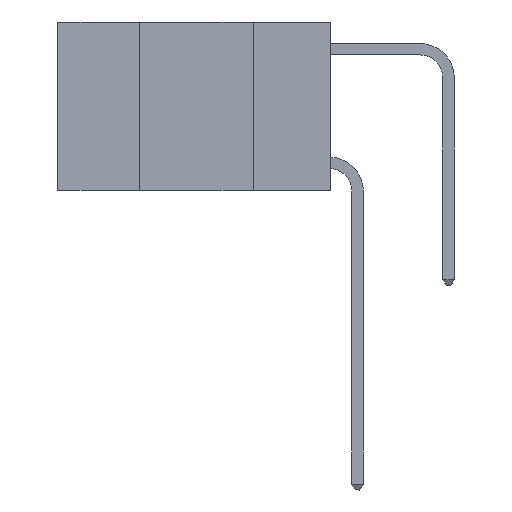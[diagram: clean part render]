
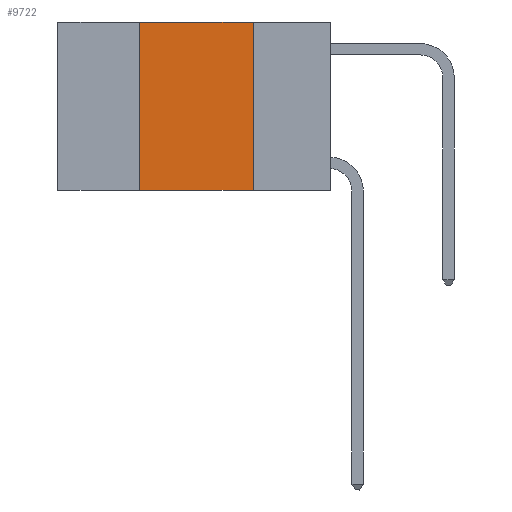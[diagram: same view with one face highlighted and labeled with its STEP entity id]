
A CAD part, left-side view. The second image highlights one B-rep face of the part: STEP entity #9722.
In plain terms, the highlighted planar face has unit normal (-1, 0, 0).
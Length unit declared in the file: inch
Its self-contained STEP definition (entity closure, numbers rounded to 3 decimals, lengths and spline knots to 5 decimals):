
#338 = ORIENTED_EDGE ( 'NONE', *, *, #16720, .T. ) ;
#473 = CARTESIAN_POINT ( 'NONE',  ( 0., 0.6, 0. ) ) ;
#1510 = CARTESIAN_POINT ( 'NONE',  ( 0., 0.6, -0.37 ) ) ;
#2065 = PLANE ( 'NONE',  #4642 ) ;
#2430 = CARTESIAN_POINT ( 'NONE',  ( 0., 0.6, 0. ) ) ;
#2546 = LINE ( 'NONE', #13820, #17581 ) ;
#3088 = EDGE_CURVE ( 'NONE', #13844, #5442, #9441, .T. ) ;
#3090 = DIRECTION ( 'NONE',  ( 0., -1., 0. ) ) ;
#4387 = VECTOR ( 'NONE', #3090, 39.37008 ) ;
#4642 = AXIS2_PLACEMENT_3D ( 'NONE', #473, #5184, #16056 ) ;
#5184 = DIRECTION ( 'NONE',  ( 1., 0., 0. ) ) ;
#5213 = CARTESIAN_POINT ( 'NONE',  ( 0., 0.42, 0. ) ) ;
#5442 = VERTEX_POINT ( 'NONE', #5213 ) ;
#6737 = CARTESIAN_POINT ( 'NONE',  ( 0., 0.42, -0.37 ) ) ;
#8958 = VECTOR ( 'NONE', #12913, 39.37008 ) ;
#9185 = EDGE_CURVE ( 'NONE', #5442, #17815, #17540, .T. ) ;
#9265 = VECTOR ( 'NONE', #13268, 39.37008 ) ;
#9441 = LINE ( 'NONE', #11352, #8958 ) ;
#9722 = ADVANCED_FACE ( 'NONE', ( #11442 ), #2065, .F. ) ;
#11352 = CARTESIAN_POINT ( 'NONE',  ( 0., 0.42, 0. ) ) ;
#11442 = FACE_OUTER_BOUND ( 'NONE', #18081, .T. ) ;
#11983 = VERTEX_POINT ( 'NONE', #18118 ) ;
#12621 = LINE ( 'NONE', #1510, #4387 ) ;
#12685 = CARTESIAN_POINT ( 'NONE',  ( 0., 0.17, 0. ) ) ;
#12913 = DIRECTION ( 'NONE',  ( 0., 0., 1. ) ) ;
#13268 = DIRECTION ( 'NONE',  ( 0., -1., 0. ) ) ;
#13820 = CARTESIAN_POINT ( 'NONE',  ( 0., 0.17, 0. ) ) ;
#13844 = VERTEX_POINT ( 'NONE', #6737 ) ;
#14162 = EDGE_CURVE ( 'NONE', #17815, #11983, #2546, .T. ) ;
#15386 = DIRECTION ( 'NONE',  ( 0., 0., -1. ) ) ;
#15918 = ORIENTED_EDGE ( 'NONE', *, *, #9185, .F. ) ;
#16056 = DIRECTION ( 'NONE',  ( 0., 0., -1. ) ) ;
#16720 = EDGE_CURVE ( 'NONE', #13844, #11983, #12621, .T. ) ;
#17540 = LINE ( 'NONE', #2430, #9265 ) ;
#17581 = VECTOR ( 'NONE', #15386, 39.37008 ) ;
#17815 = VERTEX_POINT ( 'NONE', #12685 ) ;
#18081 = EDGE_LOOP ( 'NONE', ( #18521, #15918, #19931, #338 ) ) ;
#18118 = CARTESIAN_POINT ( 'NONE',  ( 0., 0.17, -0.37 ) ) ;
#18521 = ORIENTED_EDGE ( 'NONE', *, *, #14162, .F. ) ;
#19931 = ORIENTED_EDGE ( 'NONE', *, *, #3088, .F. ) ;
